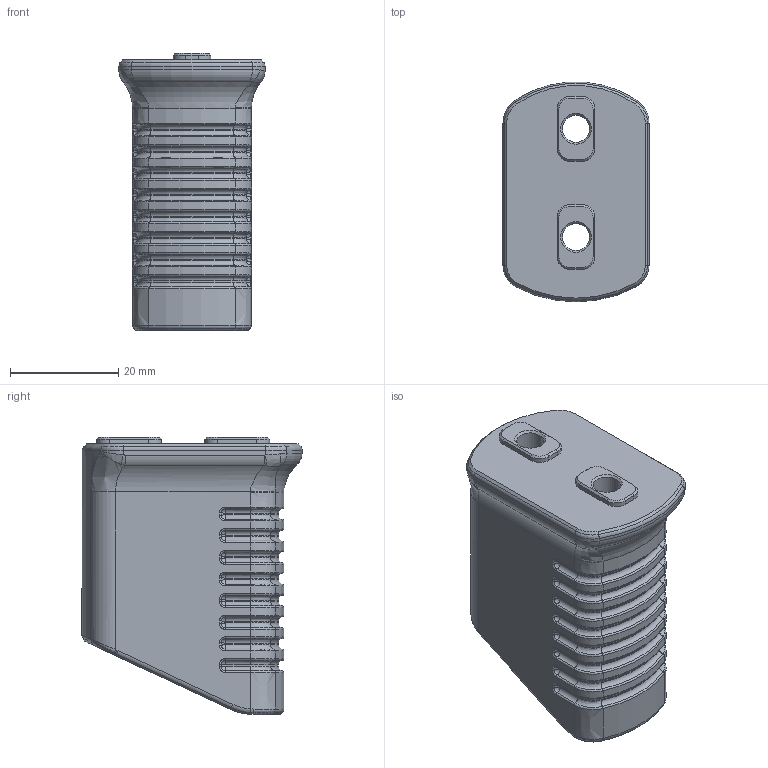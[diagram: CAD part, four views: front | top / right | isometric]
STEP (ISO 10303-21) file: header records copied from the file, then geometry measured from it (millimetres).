
FILE_DESCRIPTION(/* description */ (''),/* implementation_level */ '2;1');
FILE_NAME(/* name */ 'Micro Foregrip.step',/* time_stamp */ '2021-06-30T11:16:24-04:00',/* author */ (''),/* organization */ (''),/* preprocessor_version */ 'ST-DEVELOPER v18.1',/* originating_system */ 'Autodesk Translation Framework v10.9.0.1377',/* authorisation */ '');
FILE_SCHEMA (('AUTOMOTIVE_DESIGN { 1 0 10303 214 3 1 1 }'));
Length unit declared in the file: millimetre
Products named in the file (1): Micro Foregrip
Bounding box: 27 x 40.7 x 51.2 mm (x, y, z)
Volume: 18924.5 mm3; surface area: 10524.7 mm2
Topology: 1 solids, 1 shells, 600 faces, 1366 edges, 734 vertices
Faces by surface type: bspline 266, cylinder 171, torus 61, plane 60, cone 42
Full cylindrical faces by diameter (mm): 5 x2, 11.043 x1, 13.043 x1
Entity records: 23401 total; most frequent: CARTESIAN_POINT 11520, ORIENTED_EDGE 2652, DIRECTION 2128, EDGE_CURVE 1326, AXIS2_PLACEMENT_3D 869, VERTEX_POINT 734, EDGE_LOOP 610, FACE_OUTER_BOUND 600
